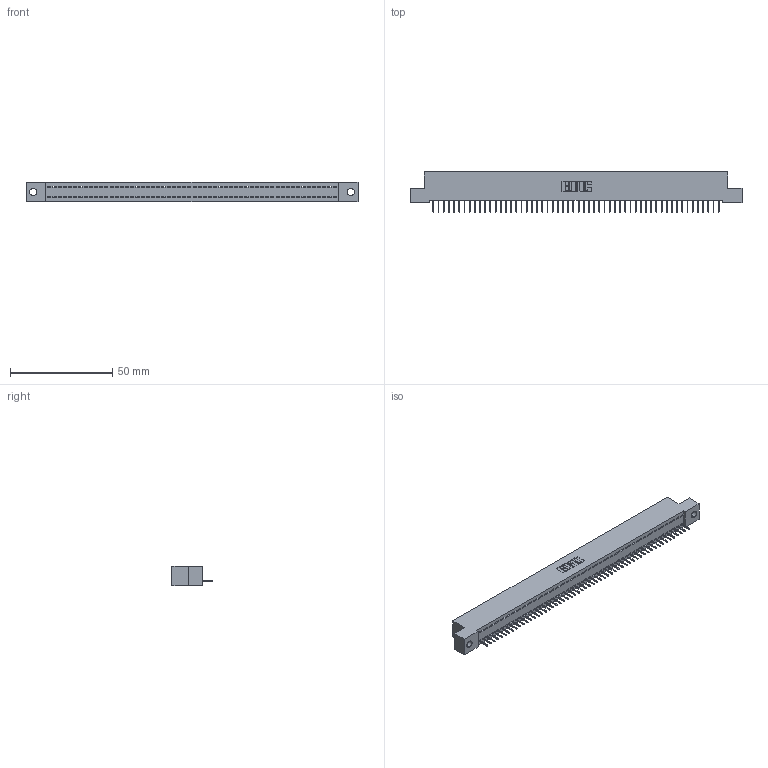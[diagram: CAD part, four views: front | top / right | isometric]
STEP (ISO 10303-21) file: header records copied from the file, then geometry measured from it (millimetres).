
FILE_DESCRIPTION (( 'STEP AP203' ), '1' );
FILE_NAME ('342-056-524-102.STEP', '2019-10-03T11:16:26', ( '' ), ( '' ), 'SwSTEP 2.0', 'SolidWorks 2016', '' );
FILE_SCHEMA (( 'CONFIG_CONTROL_DESIGN' ));
Length unit declared in the file: inch
Products named in the file (3): 345-292-001_345-293-124; 342-056-524-102; 342 Part_.128 Slot
Assembly tree (57 placements, depth 2):
  342-056-524-102
    342 Part_.128 Slot
    345-292-001_345-293-124  x56
Bounding box: 162.56 x 19.69 x 9.4 mm (x, y, z)
Volume: 14031.5 mm3; surface area: 19938.5 mm2
Topology: 57 solids, 57 shells, 3586 faces, 10391 edges, 6702 vertices
Faces by surface type: plane 2758, cylinder 828
Entity records: 32501 total; most frequent: CARTESIAN_POINT 5610, ORIENTED_EDGE 5602, DIRECTION 4705, EDGE_CURVE 2801, VECTOR 2677, LINE 2677, VERTEX_POINT 1862, AXIS2_PLACEMENT_3D 1014
